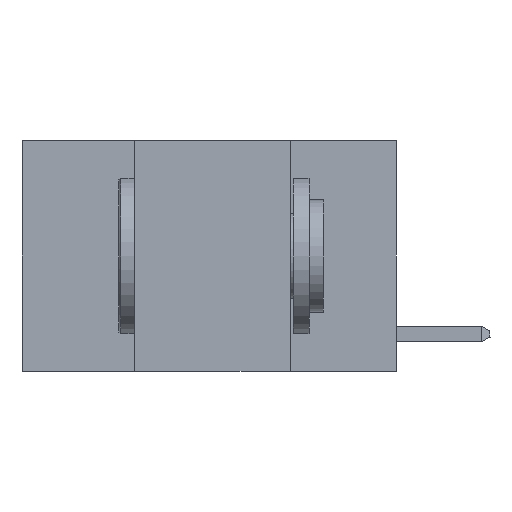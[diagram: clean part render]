
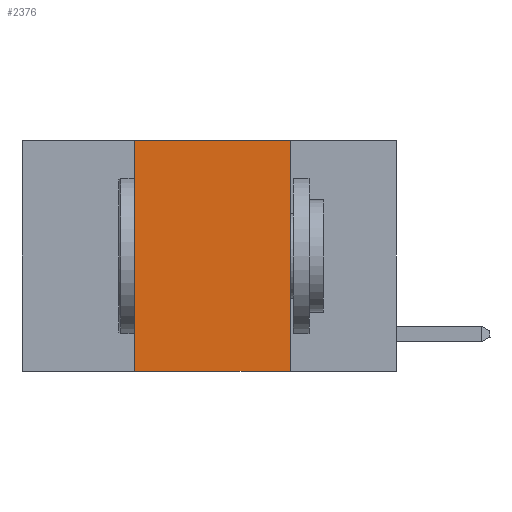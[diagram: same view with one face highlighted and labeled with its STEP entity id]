
A CAD part, left-side view. The second image highlights one B-rep face of the part: STEP entity #2376.
In plain terms, the highlighted planar face has unit normal (-1, 0, 0).
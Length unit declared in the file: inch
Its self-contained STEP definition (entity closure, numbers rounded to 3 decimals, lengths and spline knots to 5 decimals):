
#331 = CARTESIAN_POINT ( 'NONE',  ( 0., 0.17, -0.37 ) ) ;
#449 = ORIENTED_EDGE ( 'NONE', *, *, #5980, .F. ) ;
#475 = ORIENTED_EDGE ( 'NONE', *, *, #6201, .F. ) ;
#536 = ORIENTED_EDGE ( 'NONE', *, *, #2965, .F. ) ;
#550 = ORIENTED_EDGE ( 'NONE', *, *, #5026, .T. ) ;
#629 = LINE ( 'NONE', #9141, #12044 ) ;
#1772 = CARTESIAN_POINT ( 'NONE',  ( 0., 0.17, 0. ) ) ;
#1967 = VERTEX_POINT ( 'NONE', #14152 ) ;
#2125 = CARTESIAN_POINT ( 'NONE',  ( 0., 0.42, 0. ) ) ;
#2376 = ADVANCED_FACE ( 'NONE', ( #13885 ), #6736, .F. ) ;
#2769 = VECTOR ( 'NONE', #9770, 39.37008 ) ;
#2941 = VECTOR ( 'NONE', #10126, 39.37008 ) ;
#2965 = EDGE_CURVE ( 'NONE', #8950, #14276, #8749, .T. ) ;
#3395 = DIRECTION ( 'NONE',  ( 1., 0., 0. ) ) ;
#5026 = EDGE_CURVE ( 'NONE', #8950, #11481, #629, .T. ) ;
#5767 = LINE ( 'NONE', #1772, #2769 ) ;
#5980 = EDGE_CURVE ( 'NONE', #1967, #11481, #5767, .T. ) ;
#6157 = CARTESIAN_POINT ( 'NONE',  ( 0., 0.42, 0. ) ) ;
#6201 = EDGE_CURVE ( 'NONE', #14276, #1967, #11972, .T. ) ;
#6736 = PLANE ( 'NONE',  #13072 ) ;
#7986 = DIRECTION ( 'NONE',  ( 0., -1., 0. ) ) ;
#8749 = LINE ( 'NONE', #2125, #14714 ) ;
#8950 = VERTEX_POINT ( 'NONE', #10502 ) ;
#8969 = CARTESIAN_POINT ( 'NONE',  ( 0., 0.6, 0. ) ) ;
#9141 = CARTESIAN_POINT ( 'NONE',  ( 0., 0.6, -0.37 ) ) ;
#9770 = DIRECTION ( 'NONE',  ( 0., 0., -1. ) ) ;
#10126 = DIRECTION ( 'NONE',  ( 0., -1., 0. ) ) ;
#10502 = CARTESIAN_POINT ( 'NONE',  ( 0., 0.42, -0.37 ) ) ;
#11165 = DIRECTION ( 'NONE',  ( 0., 0., 1. ) ) ;
#11322 = DIRECTION ( 'NONE',  ( 0., 0., -1. ) ) ;
#11481 = VERTEX_POINT ( 'NONE', #331 ) ;
#11972 = LINE ( 'NONE', #8969, #2941 ) ;
#12044 = VECTOR ( 'NONE', #7986, 39.37008 ) ;
#13072 = AXIS2_PLACEMENT_3D ( 'NONE', #14637, #3395, #11322 ) ;
#13885 = FACE_OUTER_BOUND ( 'NONE', #13940, .T. ) ;
#13940 = EDGE_LOOP ( 'NONE', ( #449, #475, #536, #550 ) ) ;
#14152 = CARTESIAN_POINT ( 'NONE',  ( 0., 0.17, 0. ) ) ;
#14276 = VERTEX_POINT ( 'NONE', #6157 ) ;
#14637 = CARTESIAN_POINT ( 'NONE',  ( 0., 0.6, 0. ) ) ;
#14714 = VECTOR ( 'NONE', #11165, 39.37008 ) ;
